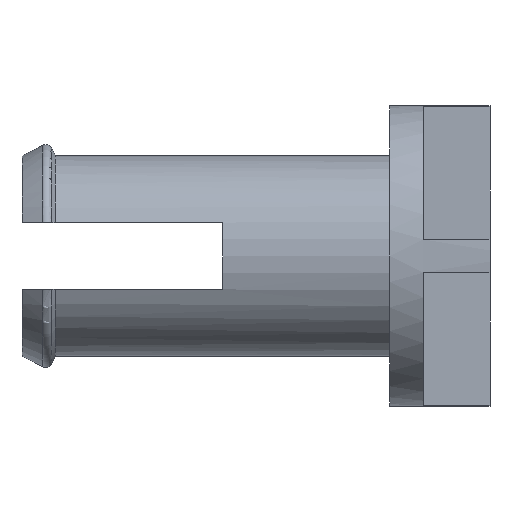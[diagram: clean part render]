
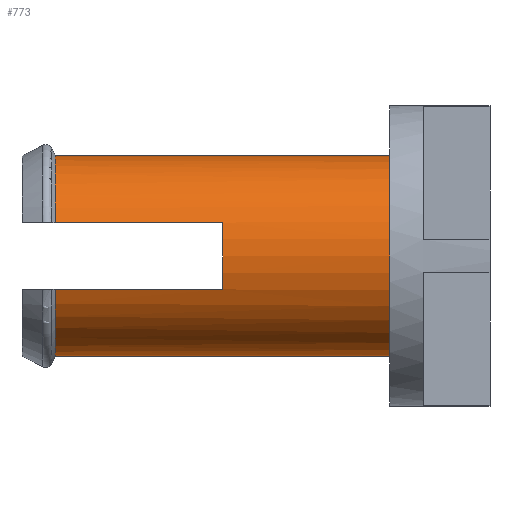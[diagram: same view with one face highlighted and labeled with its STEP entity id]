
A CAD part, left-side view. The second image highlights one B-rep face of the part: STEP entity #773.
In plain terms, the highlighted cylindrical face has radius 15 mm (diameter 30 mm), a partial arc.
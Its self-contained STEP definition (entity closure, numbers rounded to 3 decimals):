
#13 = ORIENTED_EDGE ( 'NONE', *, *, #221, .T. ) ;
#14 = ORIENTED_EDGE ( 'NONE', *, *, #42, .T. ) ;
#26 = LINE ( 'NONE', #1009, #329 ) ;
#28 = VERTEX_POINT ( 'NONE', #707 ) ;
#42 = EDGE_CURVE ( 'NONE', #1002, #1222, #1428, .T. ) ;
#44 = EDGE_CURVE ( 'NONE', #764, #28, #109, .T. ) ;
#81 = EDGE_CURVE ( 'NONE', #1204, #1088, #155, .T. ) ;
#84 = DIRECTION ( 'NONE',  ( 0., -1., 0. ) ) ;
#108 = FACE_OUTER_BOUND ( 'NONE', #1539, .T. ) ;
#109 = CIRCLE ( 'NONE', #209, 15. ) ;
#155 = CIRCLE ( 'NONE', #394, 15. ) ;
#187 = VECTOR ( 'NONE', #84, 1000. ) ;
#209 = AXIS2_PLACEMENT_3D ( 'NONE', #1114, #1313, #1129 ) ;
#221 = EDGE_CURVE ( 'NONE', #1373, #645, #1235, .T. ) ;
#224 = EDGE_CURVE ( 'NONE', #1204, #1373, #893, .T. ) ;
#282 = CARTESIAN_POINT ( 'NONE',  ( 0., 55., -15. ) ) ;
#295 = ORIENTED_EDGE ( 'NONE', *, *, #44, .F. ) ;
#328 = AXIS2_PLACEMENT_3D ( 'NONE', #652, #958, #1540 ) ;
#329 = VECTOR ( 'NONE', #359, 1000. ) ;
#341 = CARTESIAN_POINT ( 'NONE',  ( -14.142, 50., 5. ) ) ;
#344 = CARTESIAN_POINT ( 'NONE',  ( -14.142, 25., -5. ) ) ;
#345 = CARTESIAN_POINT ( 'NONE',  ( 0., 55., 0. ) ) ;
#359 = DIRECTION ( 'NONE',  ( 0., 1., 0. ) ) ;
#394 = AXIS2_PLACEMENT_3D ( 'NONE', #920, #864, #843 ) ;
#441 = AXIS2_PLACEMENT_3D ( 'NONE', #882, #669, #503 ) ;
#492 = ORIENTED_EDGE ( 'NONE', *, *, #224, .T. ) ;
#503 = DIRECTION ( 'NONE',  ( 0., 0., 1. ) ) ;
#570 = CARTESIAN_POINT ( 'NONE',  ( -14.142, 55., 5. ) ) ;
#582 = CARTESIAN_POINT ( 'NONE',  ( -14.142, 25., 5. ) ) ;
#645 = VERTEX_POINT ( 'NONE', #995 ) ;
#652 = CARTESIAN_POINT ( 'NONE',  ( 0., 25., 0. ) ) ;
#669 = DIRECTION ( 'NONE',  ( 0., 1., 0. ) ) ;
#707 = CARTESIAN_POINT ( 'NONE',  ( 0., 50., 15. ) ) ;
#739 = CYLINDRICAL_SURFACE ( 'NONE', #1444, 15. ) ;
#764 = VERTEX_POINT ( 'NONE', #341 ) ;
#773 = ADVANCED_FACE ( 'NONE', ( #108 ), #739, .T. ) ;
#843 = DIRECTION ( 'NONE',  ( 0., 0., 1. ) ) ;
#847 = CARTESIAN_POINT ( 'NONE',  ( 0., 50., -15. ) ) ;
#864 = DIRECTION ( 'NONE',  ( 0., 1., 0. ) ) ;
#882 = CARTESIAN_POINT ( 'NONE',  ( 0., 0., 0. ) ) ;
#893 = LINE ( 'NONE', #282, #1490 ) ;
#912 = LINE ( 'NONE', #570, #1506 ) ;
#920 = CARTESIAN_POINT ( 'NONE',  ( 0., 50., 0. ) ) ;
#948 = ORIENTED_EDGE ( 'NONE', *, *, #1202, .F. ) ;
#958 = DIRECTION ( 'NONE',  ( 0., -1., 0. ) ) ;
#985 = DIRECTION ( 'NONE',  ( 0., -1., 0. ) ) ;
#995 = CARTESIAN_POINT ( 'NONE',  ( 0., 0., 15. ) ) ;
#1000 = DIRECTION ( 'NONE',  ( 0., -1., 0. ) ) ;
#1002 = VERTEX_POINT ( 'NONE', #582 ) ;
#1004 = ORIENTED_EDGE ( 'NONE', *, *, #81, .F. ) ;
#1009 = CARTESIAN_POINT ( 'NONE',  ( -14.142, 55., -5. ) ) ;
#1012 = CARTESIAN_POINT ( 'NONE',  ( 0., 0., -15. ) ) ;
#1049 = ORIENTED_EDGE ( 'NONE', *, *, #1304, .T. ) ;
#1088 = VERTEX_POINT ( 'NONE', #1309 ) ;
#1103 = ORIENTED_EDGE ( 'NONE', *, *, #1133, .F. ) ;
#1114 = CARTESIAN_POINT ( 'NONE',  ( 0., 50., 0. ) ) ;
#1129 = DIRECTION ( 'NONE',  ( 0., 0., 1. ) ) ;
#1133 = EDGE_CURVE ( 'NONE', #1002, #764, #912, .T. ) ;
#1137 = LINE ( 'NONE', #1552, #187 ) ;
#1147 = DIRECTION ( 'NONE',  ( 0., 0., -1. ) ) ;
#1202 = EDGE_CURVE ( 'NONE', #28, #645, #1137, .T. ) ;
#1204 = VERTEX_POINT ( 'NONE', #847 ) ;
#1222 = VERTEX_POINT ( 'NONE', #344 ) ;
#1235 = CIRCLE ( 'NONE', #441, 15. ) ;
#1304 = EDGE_CURVE ( 'NONE', #1222, #1088, #26, .T. ) ;
#1309 = CARTESIAN_POINT ( 'NONE',  ( -14.142, 50., -5. ) ) ;
#1313 = DIRECTION ( 'NONE',  ( 0., 1., 0. ) ) ;
#1373 = VERTEX_POINT ( 'NONE', #1012 ) ;
#1428 = CIRCLE ( 'NONE', #328, 15. ) ;
#1444 = AXIS2_PLACEMENT_3D ( 'NONE', #345, #985, #1147 ) ;
#1490 = VECTOR ( 'NONE', #1000, 1000. ) ;
#1506 = VECTOR ( 'NONE', #1538, 1000. ) ;
#1538 = DIRECTION ( 'NONE',  ( 0., 1., 0. ) ) ;
#1539 = EDGE_LOOP ( 'NONE', ( #948, #295, #1103, #14, #1049, #1004, #492, #13 ) ) ;
#1540 = DIRECTION ( 'NONE',  ( 0., 0., -1. ) ) ;
#1552 = CARTESIAN_POINT ( 'NONE',  ( 0., 55., 15. ) ) ;
